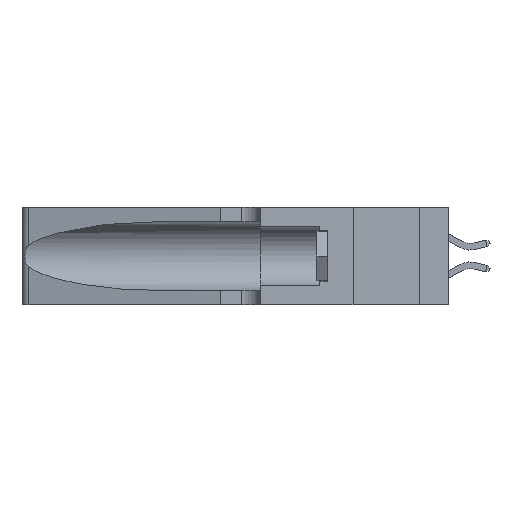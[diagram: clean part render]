
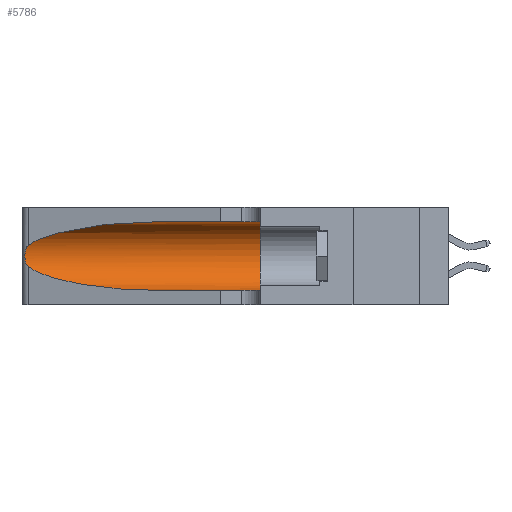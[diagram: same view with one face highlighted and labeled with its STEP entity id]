
A CAD part, left-side view. The second image highlights one B-rep face of the part: STEP entity #5786.
In plain terms, the highlighted cylindrical face has radius 3.308 mm (diameter 6.617 mm), a partial arc.
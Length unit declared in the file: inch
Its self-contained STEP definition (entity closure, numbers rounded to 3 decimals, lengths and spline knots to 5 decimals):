
#194 = CARTESIAN_POINT ( 'NONE',  ( 0.25487, 1.22718, 0.22369 ) ) ;
#281 = VERTEX_POINT ( 'NONE', #10372 ) ;
#898 = CARTESIAN_POINT ( 'NONE',  ( 0.1305, 0.35, 0.05475 ) ) ;
#907 = CARTESIAN_POINT ( 'NONE',  ( 0.1305, 1.61858, 0.185 ) ) ;
#1428 = CARTESIAN_POINT ( 'NONE',  ( 0.25555, 1.22994, 0.2215 ) ) ;
#2357 = EDGE_CURVE ( 'NONE', #6186, #23476, #3498, .T. ) ;
#2397 = EDGE_CURVE ( 'NONE', #20273, #6186, #11837, .T. ) ;
#2611 = FACE_OUTER_BOUND ( 'NONE', #15681, .T. ) ;
#2838 = DIRECTION ( 'NONE',  ( 0., 0., -1. ) ) ;
#3018 = CARTESIAN_POINT ( 'NONE',  ( 0.25487, 1.22718, 0.22369 ) ) ;
#3486 = CARTESIAN_POINT ( 'NONE',  ( 0.1305, 0.72297, 0.05475 ) ) ;
#3498 = B_SPLINE_CURVE_WITH_KNOTS ( 'NONE', 3,
 ( #3018, #1428, #4888, #12751, #13015, #12988, #12955, #12695, #23650, #4732, #8706, #6757, #8115, #21357 ),
 .UNSPECIFIED., .F., .F.,
 ( 4, 2, 2, 2, 2, 2, 4 ),
 ( 0., 0.00027, 0.00053, 0.00107, 0.0016, 0.00187, 0.00214 ),
 .UNSPECIFIED. ) ;
#4155 = CARTESIAN_POINT ( 'NONE',  ( 0.1305, 0.72297, 0.31525 ) ) ;
#4346 = CIRCLE ( 'NONE', #6190, 0.13025 ) ;
#4604 = CARTESIAN_POINT ( 'NONE',  ( 0.18966, 0.96281, 0.05475 ) ) ;
#4732 = CARTESIAN_POINT ( 'NONE',  ( 0.25856, 1.23593, 0.16098 ) ) ;
#4888 = CARTESIAN_POINT ( 'NONE',  ( 0.25639, 1.23184, 0.21858 ) ) ;
#5674 = EDGE_CURVE ( 'NONE', #23476, #20547, #16502, .T. ) ;
#5786 = ADVANCED_FACE ( 'NONE', ( #2611 ), #11526, .F. ) ;
#6186 = VERTEX_POINT ( 'NONE', #194 ) ;
#6190 = AXIS2_PLACEMENT_3D ( 'NONE', #20149, #9441, #21915 ) ;
#6540 = LINE ( 'NONE', #18771, #20386 ) ;
#6687 = DIRECTION ( 'NONE',  ( 0., -1., 0. ) ) ;
#6725 = ORIENTED_EDGE ( 'NONE', *, *, #15454, .T. ) ;
#6757 = CARTESIAN_POINT ( 'NONE',  ( 0.25639, 1.23186, 0.15144 ) ) ;
#7065 = EDGE_CURVE ( 'NONE', #281, #8191, #4346, .T. ) ;
#7967 = CARTESIAN_POINT ( 'NONE',  ( 0.25487, 1.22718, 0.22369 ) ) ;
#8115 = CARTESIAN_POINT ( 'NONE',  ( 0.25555, 1.22993, 0.14849 ) ) ;
#8191 = VERTEX_POINT ( 'NONE', #898 ) ;
#8706 = CARTESIAN_POINT ( 'NONE',  ( 0.25789, 1.23486, 0.15765 ) ) ;
#9076 = ORIENTED_EDGE ( 'NONE', *, *, #7065, .F. ) ;
#9325 = CARTESIAN_POINT ( 'NONE',  ( 0.2373, 1.15595, 0.28018 ) ) ;
#9441 = DIRECTION ( 'NONE',  ( 0., 1., 0. ) ) ;
#10167 = CARTESIAN_POINT ( 'NONE',  ( 0.1305, 1.61858, 0.05475 ) ) ;
#10372 = CARTESIAN_POINT ( 'NONE',  ( 0.1305, 0.35, 0.31525 ) ) ;
#11526 = CYLINDRICAL_SURFACE ( 'NONE', #11857, 0.13025 ) ;
#11837 =( BOUNDED_CURVE ( )  B_SPLINE_CURVE ( 3, ( #4155, #23051, #9325, #7967 ),
 .UNSPECIFIED., .F., .T. ) 
 B_SPLINE_CURVE_WITH_KNOTS ( ( 4, 4 ),
 ( 1.5708, 2.84003 ),
 .UNSPECIFIED. ) 
 CURVE ( )  GEOMETRIC_REPRESENTATION_ITEM ( )  RATIONAL_B_SPLINE_CURVE ( ( 1., 0.87, 0.87, 1. ) ) 
 REPRESENTATION_ITEM ( '' )  );
#11857 = AXIS2_PLACEMENT_3D ( 'NONE', #907, #6687, #2838 ) ;
#12695 = CARTESIAN_POINT ( 'NONE',  ( 0.26075, 1.23896, 0.178 ) ) ;
#12751 = CARTESIAN_POINT ( 'NONE',  ( 0.25787, 1.23484, 0.2124 ) ) ;
#12955 = CARTESIAN_POINT ( 'NONE',  ( 0.26075, 1.23896, 0.19203 ) ) ;
#12988 = CARTESIAN_POINT ( 'NONE',  ( 0.26018, 1.23835, 0.19895 ) ) ;
#13015 = CARTESIAN_POINT ( 'NONE',  ( 0.25854, 1.2359, 0.20912 ) ) ;
#13885 = CARTESIAN_POINT ( 'NONE',  ( 0.25487, 1.22718, 0.14631 ) ) ;
#13938 = CARTESIAN_POINT ( 'NONE',  ( 0.1305, 0.72297, 0.31525 ) ) ;
#14434 = CARTESIAN_POINT ( 'NONE',  ( 0.25487, 1.22718, 0.14631 ) ) ;
#15454 = EDGE_CURVE ( 'NONE', #20547, #8191, #22044, .T. ) ;
#15647 = CARTESIAN_POINT ( 'NONE',  ( 0.2373, 1.15595, 0.08982 ) ) ;
#15681 = EDGE_LOOP ( 'NONE', ( #23234, #21351, #22491, #6725, #9076, #16816 ) ) ;
#16502 =( BOUNDED_CURVE ( )  B_SPLINE_CURVE ( 3, ( #13885, #15647, #4604, #17415 ),
 .UNSPECIFIED., .F., .T. ) 
 B_SPLINE_CURVE_WITH_KNOTS ( ( 4, 4 ),
 ( 3.44316, 4.71239 ),
 .UNSPECIFIED. ) 
 CURVE ( )  GEOMETRIC_REPRESENTATION_ITEM ( )  RATIONAL_B_SPLINE_CURVE ( ( 1., 0.87, 0.87, 1. ) ) 
 REPRESENTATION_ITEM ( '' )  );
#16816 = ORIENTED_EDGE ( 'NONE', *, *, #23157, .F. ) ;
#17415 = CARTESIAN_POINT ( 'NONE',  ( 0.1305, 0.72297, 0.05475 ) ) ;
#17932 = VECTOR ( 'NONE', #20828, 39.37008 ) ;
#18771 = CARTESIAN_POINT ( 'NONE',  ( 0.1305, 1.61858, 0.31525 ) ) ;
#20149 = CARTESIAN_POINT ( 'NONE',  ( 0.1305, 0.35, 0.185 ) ) ;
#20273 = VERTEX_POINT ( 'NONE', #13938 ) ;
#20386 = VECTOR ( 'NONE', #20555, 39.37008 ) ;
#20547 = VERTEX_POINT ( 'NONE', #3486 ) ;
#20555 = DIRECTION ( 'NONE',  ( 0., -1., 0. ) ) ;
#20828 = DIRECTION ( 'NONE',  ( 0., -1., 0. ) ) ;
#21351 = ORIENTED_EDGE ( 'NONE', *, *, #2357, .T. ) ;
#21357 = CARTESIAN_POINT ( 'NONE',  ( 0.25487, 1.22718, 0.14631 ) ) ;
#21915 = DIRECTION ( 'NONE',  ( 0., 0., 1. ) ) ;
#22044 = LINE ( 'NONE', #10167, #17932 ) ;
#22491 = ORIENTED_EDGE ( 'NONE', *, *, #5674, .T. ) ;
#23051 = CARTESIAN_POINT ( 'NONE',  ( 0.18966, 0.96281, 0.31525 ) ) ;
#23157 = EDGE_CURVE ( 'NONE', #20273, #281, #6540, .T. ) ;
#23234 = ORIENTED_EDGE ( 'NONE', *, *, #2397, .T. ) ;
#23476 = VERTEX_POINT ( 'NONE', #14434 ) ;
#23650 = CARTESIAN_POINT ( 'NONE',  ( 0.26017, 1.23833, 0.17102 ) ) ;
